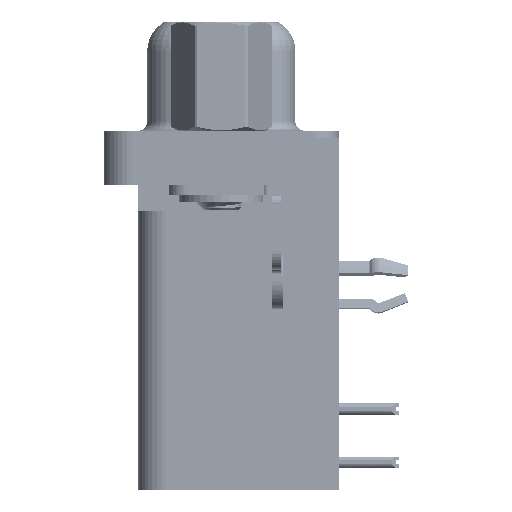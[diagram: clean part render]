
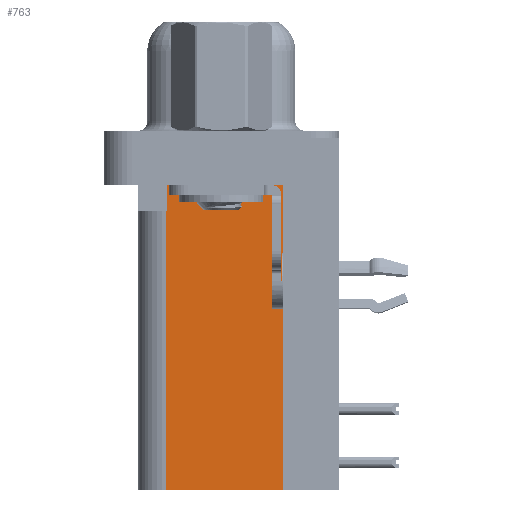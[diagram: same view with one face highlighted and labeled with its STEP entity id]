
A CAD part, left-side view. The second image highlights one B-rep face of the part: STEP entity #763.
In plain terms, the highlighted planar face has unit normal (-1, 0, 0).
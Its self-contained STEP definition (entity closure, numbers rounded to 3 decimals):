
#365 = DIRECTION ( 'NONE',  ( 0., 0., 1. ) ) ;
#763 = ADVANCED_FACE ( 'NONE', ( #20509 ), #6904, .F. ) ;
#1033 = VECTOR ( 'NONE', #365, 1000. ) ;
#1106 = CARTESIAN_POINT ( 'NONE',  ( 3.79, 2.925, -18.76 ) ) ;
#1108 = LINE ( 'NONE', #3844, #1395 ) ;
#1236 = LINE ( 'NONE', #20633, #1033 ) ;
#1395 = VECTOR ( 'NONE', #7209, 1000. ) ;
#2755 = VECTOR ( 'NONE', #11767, 1000. ) ;
#2883 = LINE ( 'NONE', #41280, #2755 ) ;
#3844 = CARTESIAN_POINT ( 'NONE',  ( 3.79, -3.295, -18.76 ) ) ;
#6904 = PLANE ( 'NONE',  #14186 ) ;
#7209 = DIRECTION ( 'NONE',  ( 0., 1., 0. ) ) ;
#8581 = VECTOR ( 'NONE', #38292, 1000. ) ;
#8682 = CARTESIAN_POINT ( 'NONE',  ( 3.79, 2.925, -3.9 ) ) ;
#8714 = LINE ( 'NONE', #22001, #8581 ) ;
#8835 = DIRECTION ( 'NONE',  ( 1., 0., 0. ) ) ;
#9177 = CARTESIAN_POINT ( 'NONE',  ( 3.79, -3.295, -18.76 ) ) ;
#11206 = CARTESIAN_POINT ( 'NONE',  ( 3.79, -3.295, -2.5 ) ) ;
#11767 = DIRECTION ( 'NONE',  ( 0., 1., 0. ) ) ;
#12431 = EDGE_CURVE ( 'NONE', #38941, #21246, #8714, .T. ) ;
#14186 = AXIS2_PLACEMENT_3D ( 'NONE', #9177, #8835, #42246 ) ;
#14367 = ORIENTED_EDGE ( 'NONE', *, *, #12431, .T. ) ;
#19735 = ORIENTED_EDGE ( 'NONE', *, *, #34514, .T. ) ;
#20005 = DIRECTION ( 'NONE',  ( 0., 0., 1. ) ) ;
#20509 = FACE_OUTER_BOUND ( 'NONE', #41158, .T. ) ;
#20616 = VERTEX_POINT ( 'NONE', #26828 ) ;
#20633 = CARTESIAN_POINT ( 'NONE',  ( 3.79, -3.295, -18.76 ) ) ;
#21246 = VERTEX_POINT ( 'NONE', #30581 ) ;
#21877 = EDGE_CURVE ( 'NONE', #20616, #30068, #2883, .T. ) ;
#22001 = CARTESIAN_POINT ( 'NONE',  ( 3.79, -3.295, -2.5 ) ) ;
#22027 = VECTOR ( 'NONE', #34057, 1000. ) ;
#22622 = LINE ( 'NONE', #42853, #22027 ) ;
#22882 = EDGE_CURVE ( 'NONE', #38132, #30068, #28067, .T. ) ;
#23171 = ORIENTED_EDGE ( 'NONE', *, *, #21877, .T. ) ;
#23342 = ORIENTED_EDGE ( 'NONE', *, *, #22882, .F. ) ;
#26828 = CARTESIAN_POINT ( 'NONE',  ( 3.79, 2.895, -3.9 ) ) ;
#27453 = VECTOR ( 'NONE', #20005, 1000. ) ;
#28067 = LINE ( 'NONE', #36183, #27453 ) ;
#30068 = VERTEX_POINT ( 'NONE', #8682 ) ;
#30119 = VERTEX_POINT ( 'NONE', #41954 ) ;
#30581 = CARTESIAN_POINT ( 'NONE',  ( 3.79, 2.895, -2.5 ) ) ;
#30757 = ORIENTED_EDGE ( 'NONE', *, *, #31319, .F. ) ;
#31309 = EDGE_CURVE ( 'NONE', #30119, #38941, #1236, .T. ) ;
#31319 = EDGE_CURVE ( 'NONE', #30119, #38132, #1108, .T. ) ;
#34057 = DIRECTION ( 'NONE',  ( 0., 0., -1. ) ) ;
#34514 = EDGE_CURVE ( 'NONE', #21246, #20616, #22622, .T. ) ;
#34782 = ORIENTED_EDGE ( 'NONE', *, *, #31309, .T. ) ;
#36183 = CARTESIAN_POINT ( 'NONE',  ( 3.79, 2.925, -18.76 ) ) ;
#38132 = VERTEX_POINT ( 'NONE', #1106 ) ;
#38292 = DIRECTION ( 'NONE',  ( 0., 1., 0. ) ) ;
#38941 = VERTEX_POINT ( 'NONE', #11206 ) ;
#41158 = EDGE_LOOP ( 'NONE', ( #14367, #19735, #23171, #23342, #30757, #34782 ) ) ;
#41280 = CARTESIAN_POINT ( 'NONE',  ( 3.79, 0., -3.9 ) ) ;
#41954 = CARTESIAN_POINT ( 'NONE',  ( 3.79, -3.295, -18.76 ) ) ;
#42246 = DIRECTION ( 'NONE',  ( 0., 1., 0. ) ) ;
#42853 = CARTESIAN_POINT ( 'NONE',  ( 3.79, 2.895, -3.9 ) ) ;
